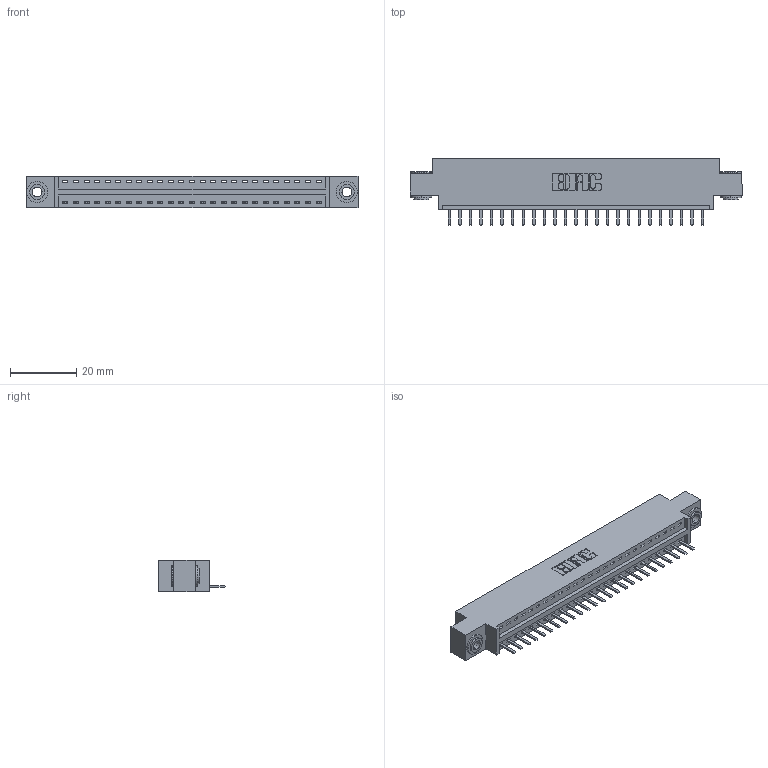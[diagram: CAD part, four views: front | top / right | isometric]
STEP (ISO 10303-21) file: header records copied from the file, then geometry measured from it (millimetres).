
FILE_DESCRIPTION (( 'STEP AP203' ), '1' );
FILE_NAME ('346-025-520-603.STEP', '2022-05-06T00:11:33', ( '' ), ( '' ), 'SwSTEP 2.0', 'SolidWorks 2020', '' );
FILE_SCHEMA (( 'CONFIG_CONTROL_DESIGN' ));
Length unit declared in the file: inch
Products named in the file (4): 345-250-002_345-250-002-102; 346-025-520-603; 346 Part_0.170 Offset - 0.156 Dia-TH; 345-292-001_345-293-120
Assembly tree (28 placements, depth 2):
  346-025-520-603
    346 Part_0.170 Offset - 0.156 Dia-TH
    345-292-001_345-293-120  x25
    345-250-002_345-250-002-102  x2
Bounding box: 99.95 x 20.02 x 9.4 mm (x, y, z)
Volume: 9225 mm3; surface area: 11518.3 mm2
Topology: 28 solids, 28 shells, 1728 faces, 5053 edges, 3298 vertices
Faces by surface type: plane 1154, cylinder 566, cone 8
Entity records: 19116 total; most frequent: CARTESIAN_POINT 3276, ORIENTED_EDGE 3214, DIRECTION 2927, EDGE_CURVE 1607, VECTOR 1347, LINE 1347, VERTEX_POINT 1066, AXIS2_PLACEMENT_3D 790
